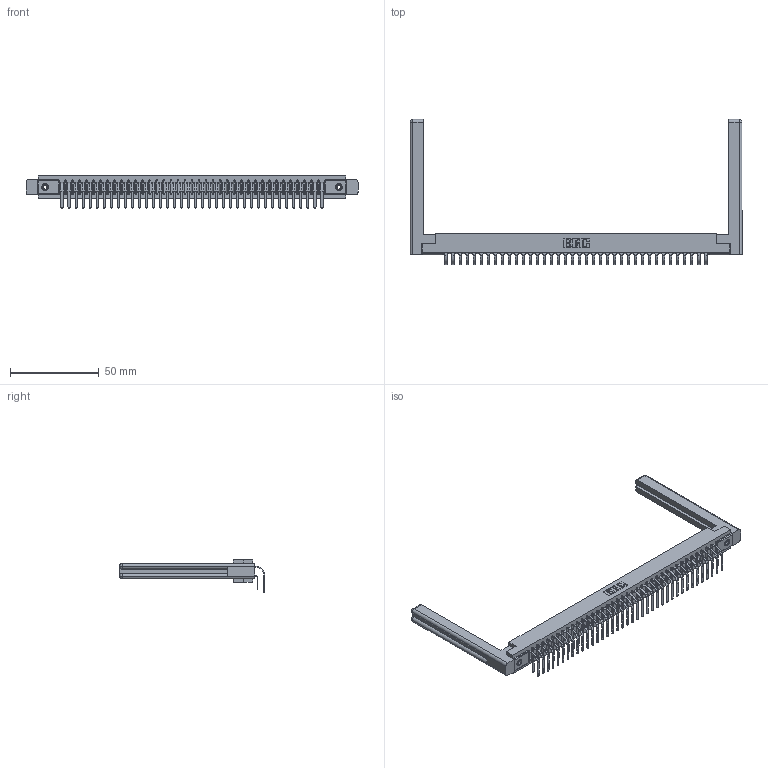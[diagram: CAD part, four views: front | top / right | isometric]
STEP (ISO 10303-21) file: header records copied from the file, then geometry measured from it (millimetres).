
FILE_DESCRIPTION (( 'STEP AP203' ), '1' );
FILE_NAME ('357-076-559-258.STEP', '2022-07-08T20:39:41', ( '' ), ( '' ), 'SwSTEP 2.0', 'SolidWorks 2020', '' );
FILE_SCHEMA (( 'CONFIG_CONTROL_DESIGN' ));
Length unit declared in the file: inch
Products named in the file (6): 357-076-559-258; 307 Part_.156 Dia Mounting Holes; 307-220-058; 345-250-001_345-250-001-102; 307-290-001_559 - 2 (Single); 307-290-001_558 559 - 1 (Single)
Assembly tree (81 placements, depth 2):
  357-076-559-258
    307 Part_.156 Dia Mounting Holes
    307-290-001_558 559 - 1 (Single)  x38
    307-290-001_559 - 2 (Single)  x38
    307-220-058  x2
    345-250-001_345-250-001-102  x2
Bounding box: 187.2 x 81.83 x 18.07 mm (x, y, z)
Volume: 27293.2 mm3; surface area: 31112.8 mm2
Topology: 81 solids, 81 shells, 4099 faces, 11469 edges, 7426 vertices
Faces by surface type: plane 2662, cylinder 1335, sphere 78, torus 12, cone 12
Entity records: 38366 total; most frequent: CARTESIAN_POINT 6299, ORIENTED_EDGE 6184, DIRECTION 6128, EDGE_CURVE 3092, VECTOR 2366, LINE 2366, VERTEX_POINT 1998, AXIS2_PLACEMENT_3D 1881
